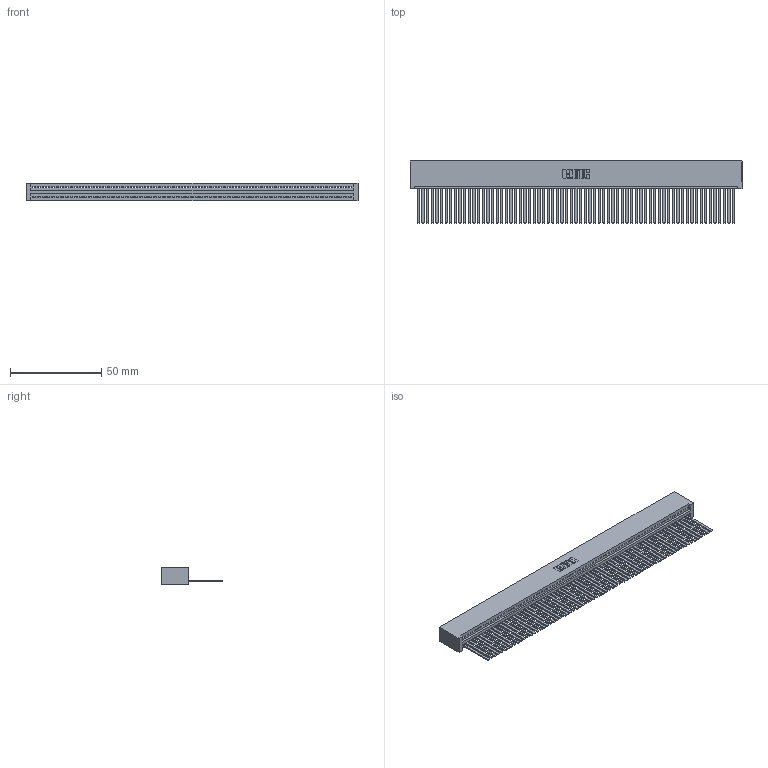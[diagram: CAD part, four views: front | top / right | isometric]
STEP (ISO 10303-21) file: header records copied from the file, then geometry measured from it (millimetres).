
FILE_DESCRIPTION (( 'STEP AP203' ), '1' );
FILE_NAME ('345-069-544-101.STEP', '2019-10-12T12:50:31', ( '' ), ( '' ), 'SwSTEP 2.0', 'SolidWorks 2016', '' );
FILE_SCHEMA (( 'CONFIG_CONTROL_DESIGN' ));
Length unit declared in the file: inch
Products named in the file (3): 345 Part_No Mounting Lugs; 345-069-544-101; 345-292-001_345-293-144
Assembly tree (70 placements, depth 2):
  345-069-544-101
    345 Part_No Mounting Lugs
    345-292-001_345-293-144  x69
Bounding box: 181.86 x 33.96 x 9.4 mm (x, y, z)
Volume: 18878.3 mm3; surface area: 28043.6 mm2
Topology: 70 solids, 70 shells, 3706 faces, 11219 edges, 7386 vertices
Faces by surface type: plane 2560, cylinder 1146
Entity records: 47835 total; most frequent: ORIENTED_EDGE 8294, CARTESIAN_POINT 8291, DIRECTION 7193, EDGE_CURVE 4147, VECTOR 3751, LINE 3751, VERTEX_POINT 2762, AXIS2_PLACEMENT_3D 1721
